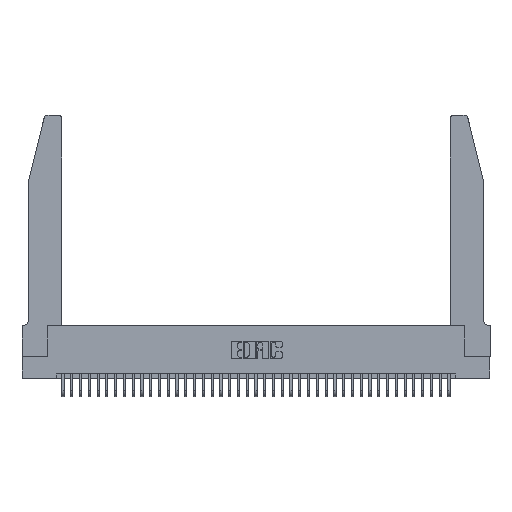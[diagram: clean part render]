
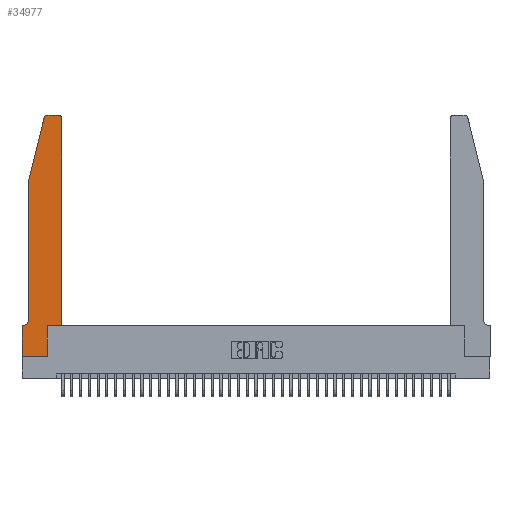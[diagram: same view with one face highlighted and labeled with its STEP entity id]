
A CAD part, top view. The second image highlights one B-rep face of the part: STEP entity #34977.
In plain terms, the highlighted planar face has unit normal (0, 0, 1).
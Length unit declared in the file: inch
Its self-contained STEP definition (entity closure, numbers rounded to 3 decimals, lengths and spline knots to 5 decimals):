
#44 = ORIENTED_EDGE ( 'NONE', *, *, #40243, .T. ) ;
#118 = ORIENTED_EDGE ( 'NONE', *, *, #11224, .T. ) ;
#757 = CARTESIAN_POINT ( 'NONE',  ( 0.0755, 0.35, 0.37 ) ) ;
#939 = CARTESIAN_POINT ( 'NONE',  ( 0.2865, 0.35, 0.37 ) ) ;
#1890 = CARTESIAN_POINT ( 'NONE',  ( 0.284, 2.75, 0.37 ) ) ;
#2136 = EDGE_CURVE ( 'NONE', #12608, #2801, #6404, .T. ) ;
#2330 = CARTESIAN_POINT ( 'NONE',  ( 0., 0., 0.37 ) ) ;
#2625 = DIRECTION ( 'NONE',  ( 0., -1., 0. ) ) ;
#2801 = VERTEX_POINT ( 'NONE', #33554 ) ;
#2832 = VECTOR ( 'NONE', #33975, 39.37008 ) ;
#5162 = CARTESIAN_POINT ( 'NONE',  ( 0.0755, 2., 0.37 ) ) ;
#6372 = EDGE_CURVE ( 'NONE', #10322, #16727, #36225, .T. ) ;
#6404 = LINE ( 'NONE', #37515, #31408 ) ;
#6511 = VECTOR ( 'NONE', #23060, 39.37008 ) ;
#7188 = CARTESIAN_POINT ( 'NONE',  ( 0.0755, 2., 0.37 ) ) ;
#7669 = LINE ( 'NONE', #2330, #35153 ) ;
#8680 = DIRECTION ( 'NONE',  ( 1., 0., 0. ) ) ;
#9171 = VERTEX_POINT ( 'NONE', #24480 ) ;
#9280 = DIRECTION ( 'NONE',  ( 0., 0., -1. ) ) ;
#9764 = EDGE_LOOP ( 'NONE', ( #24207, #118, #27873, #29257, #39053, #44, #20807, #10522, #32796, #18985, #34680, #21698 ) ) ;
#9779 = LINE ( 'NONE', #27875, #24731 ) ;
#10204 = AXIS2_PLACEMENT_3D ( 'NONE', #27847, #27708, #8680 ) ;
#10322 = VERTEX_POINT ( 'NONE', #11757 ) ;
#10522 = ORIENTED_EDGE ( 'NONE', *, *, #35061, .T. ) ;
#11224 = EDGE_CURVE ( 'NONE', #38254, #21556, #25684, .T. ) ;
#11492 = VERTEX_POINT ( 'NONE', #36402 ) ;
#11528 = EDGE_CURVE ( 'NONE', #27020, #20467, #20231, .T. ) ;
#11693 = CARTESIAN_POINT ( 'NONE',  ( 0.0055, 0.35, 0.37 ) ) ;
#11757 = CARTESIAN_POINT ( 'NONE',  ( 0.0755, 0.42, 0.37 ) ) ;
#12043 = LINE ( 'NONE', #757, #6511 ) ;
#12509 = DIRECTION ( 'NONE',  ( 0., 0., 1. ) ) ;
#12608 = VERTEX_POINT ( 'NONE', #13570 ) ;
#13570 = CARTESIAN_POINT ( 'NONE',  ( 0.2865, 0.35, 0.37 ) ) ;
#14084 = DIRECTION ( 'NONE',  ( -1., 0., 0. ) ) ;
#14192 = CARTESIAN_POINT ( 'NONE',  ( 0.4505, 2.72, 0.37 ) ) ;
#14383 = VERTEX_POINT ( 'NONE', #23230 ) ;
#14406 = VECTOR ( 'NONE', #39241, 39.37008 ) ;
#14563 = LINE ( 'NONE', #21612, #28060 ) ;
#15510 = EDGE_CURVE ( 'NONE', #21556, #16330, #19895, .T. ) ;
#16219 = EDGE_CURVE ( 'NONE', #14383, #9171, #21413, .T. ) ;
#16330 = VERTEX_POINT ( 'NONE', #5162 ) ;
#16549 = CARTESIAN_POINT ( 'NONE',  ( 0.25487, 2.72718, 0.37 ) ) ;
#16727 = VERTEX_POINT ( 'NONE', #11693 ) ;
#17014 = CARTESIAN_POINT ( 'NONE',  ( 0., 0., 0.37 ) ) ;
#18244 = DIRECTION ( 'NONE',  ( -1., 0., 0. ) ) ;
#18829 = VECTOR ( 'NONE', #14084, 39.37008 ) ;
#18985 = ORIENTED_EDGE ( 'NONE', *, *, #2136, .T. ) ;
#19895 = LINE ( 'NONE', #7188, #14406 ) ;
#20231 = CIRCLE ( 'NONE', #22296, 0.03 ) ;
#20467 = VERTEX_POINT ( 'NONE', #23410 ) ;
#20798 = LINE ( 'NONE', #939, #2832 ) ;
#20807 = ORIENTED_EDGE ( 'NONE', *, *, #16219, .T. ) ;
#21413 = LINE ( 'NONE', #17014, #31410 ) ;
#21556 = VERTEX_POINT ( 'NONE', #16549 ) ;
#21607 = DIRECTION ( 'NONE',  ( 1., 0., 0. ) ) ;
#21612 = CARTESIAN_POINT ( 'NONE',  ( 0.0755, 2., 0.37 ) ) ;
#21698 = ORIENTED_EDGE ( 'NONE', *, *, #11528, .T. ) ;
#22296 = AXIS2_PLACEMENT_3D ( 'NONE', #31542, #32526, #39826 ) ;
#23060 = DIRECTION ( 'NONE',  ( -1., 0., 0. ) ) ;
#23230 = CARTESIAN_POINT ( 'NONE',  ( 0., 0.35, 0.37 ) ) ;
#23410 = CARTESIAN_POINT ( 'NONE',  ( 0.4205, 2.75, 0.37 ) ) ;
#23814 = EDGE_CURVE ( 'NONE', #11492, #12608, #20798, .T. ) ;
#24207 = ORIENTED_EDGE ( 'NONE', *, *, #33964, .T. ) ;
#24480 = CARTESIAN_POINT ( 'NONE',  ( 0., 0., 0.37 ) ) ;
#24731 = VECTOR ( 'NONE', #34553, 39.37008 ) ;
#24909 = DIRECTION ( 'NONE',  ( 1., 0., 0. ) ) ;
#25684 = CIRCLE ( 'NONE', #10204, 0.03 ) ;
#26881 = AXIS2_PLACEMENT_3D ( 'NONE', #28152, #12509, #24909 ) ;
#27020 = VERTEX_POINT ( 'NONE', #14192 ) ;
#27708 = DIRECTION ( 'NONE',  ( 0., 0., 1. ) ) ;
#27847 = CARTESIAN_POINT ( 'NONE',  ( 0.284, 2.72, 0.37 ) ) ;
#27873 = ORIENTED_EDGE ( 'NONE', *, *, #15510, .T. ) ;
#27875 = CARTESIAN_POINT ( 'NONE',  ( 0.4505, 0.35, 0.37 ) ) ;
#28011 = PLANE ( 'NONE',  #26881 ) ;
#28060 = VECTOR ( 'NONE', #2625, 39.37008 ) ;
#28152 = CARTESIAN_POINT ( 'NONE',  ( 0., 0.35, 0.37 ) ) ;
#28409 = CARTESIAN_POINT ( 'NONE',  ( 0.0055, 0.42, 0.37 ) ) ;
#29098 = DIRECTION ( 'NONE',  ( 1., 0., 0. ) ) ;
#29257 = ORIENTED_EDGE ( 'NONE', *, *, #39850, .T. ) ;
#29979 = DIRECTION ( 'NONE',  ( 0., -1., 0. ) ) ;
#31408 = VECTOR ( 'NONE', #21607, 39.37008 ) ;
#31410 = VECTOR ( 'NONE', #29979, 39.37008 ) ;
#31542 = CARTESIAN_POINT ( 'NONE',  ( 0.4205, 2.72, 0.37 ) ) ;
#32307 = AXIS2_PLACEMENT_3D ( 'NONE', #28409, #9280, #18244 ) ;
#32526 = DIRECTION ( 'NONE',  ( 0., 0., 1. ) ) ;
#32774 = LINE ( 'NONE', #33077, #18829 ) ;
#32796 = ORIENTED_EDGE ( 'NONE', *, *, #23814, .T. ) ;
#33077 = CARTESIAN_POINT ( 'NONE',  ( 0.2605, 2.75, 0.37 ) ) ;
#33554 = CARTESIAN_POINT ( 'NONE',  ( 0.4505, 0.35, 0.37 ) ) ;
#33964 = EDGE_CURVE ( 'NONE', #20467, #38254, #32774, .T. ) ;
#33975 = DIRECTION ( 'NONE',  ( 0., 1., 0. ) ) ;
#34553 = DIRECTION ( 'NONE',  ( 0., 1., 0. ) ) ;
#34680 = ORIENTED_EDGE ( 'NONE', *, *, #36926, .T. ) ;
#34977 = ADVANCED_FACE ( 'NONE', ( #40227 ), #28011, .T. ) ;
#35061 = EDGE_CURVE ( 'NONE', #9171, #11492, #7669, .T. ) ;
#35153 = VECTOR ( 'NONE', #29098, 39.37008 ) ;
#36225 = CIRCLE ( 'NONE', #32307, 0.07 ) ;
#36402 = CARTESIAN_POINT ( 'NONE',  ( 0.2865, 0., 0.37 ) ) ;
#36926 = EDGE_CURVE ( 'NONE', #2801, #27020, #9779, .T. ) ;
#37515 = CARTESIAN_POINT ( 'NONE',  ( 0.4505, 0.35, 0.37 ) ) ;
#38254 = VERTEX_POINT ( 'NONE', #1890 ) ;
#39053 = ORIENTED_EDGE ( 'NONE', *, *, #6372, .T. ) ;
#39241 = DIRECTION ( 'NONE',  ( -0.239, -0.971, 0. ) ) ;
#39826 = DIRECTION ( 'NONE',  ( 1., 0., 0. ) ) ;
#39850 = EDGE_CURVE ( 'NONE', #16330, #10322, #14563, .T. ) ;
#40227 = FACE_OUTER_BOUND ( 'NONE', #9764, .T. ) ;
#40243 = EDGE_CURVE ( 'NONE', #16727, #14383, #12043, .T. ) ;
